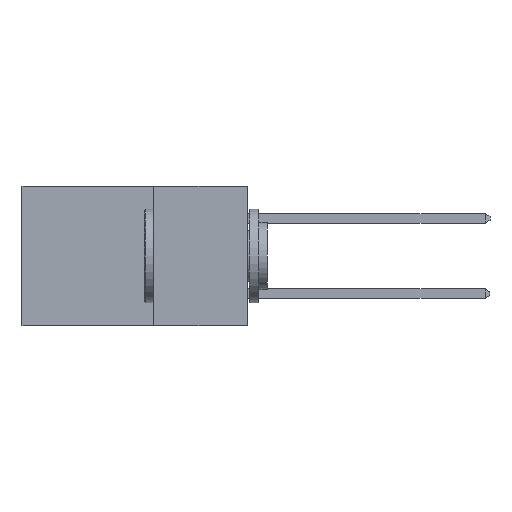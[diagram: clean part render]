
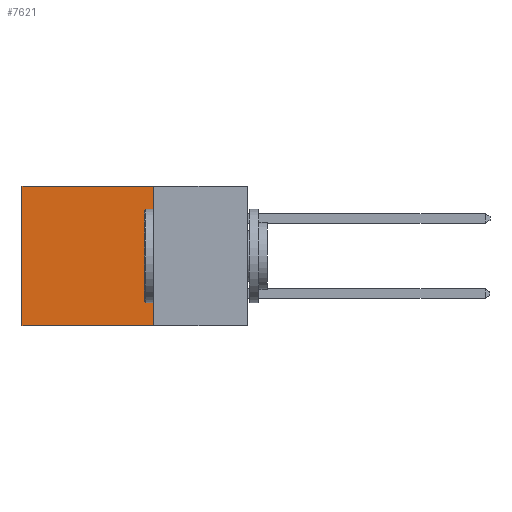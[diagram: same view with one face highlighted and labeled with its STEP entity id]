
A CAD part, left-side view. The second image highlights one B-rep face of the part: STEP entity #7621.
In plain terms, the highlighted planar face has unit normal (-1, 0, 0).
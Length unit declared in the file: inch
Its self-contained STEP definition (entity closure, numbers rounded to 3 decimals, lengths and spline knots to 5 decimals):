
#646 = EDGE_CURVE ( 'NONE', #6985, #10726, #9154, .T. ) ;
#1405 = VERTEX_POINT ( 'NONE', #12467 ) ;
#1589 = DIRECTION ( 'NONE',  ( 1., 0., 0. ) ) ;
#2355 = ORIENTED_EDGE ( 'NONE', *, *, #13315, .F. ) ;
#2408 = CARTESIAN_POINT ( 'NONE',  ( 0.298, 0.25, -0.37 ) ) ;
#2529 = CARTESIAN_POINT ( 'NONE',  ( 0.298, 0.25, 0. ) ) ;
#3327 = CARTESIAN_POINT ( 'NONE',  ( 0.298, 0.25, -0.37 ) ) ;
#3564 = VECTOR ( 'NONE', #13073, 39.37008 ) ;
#3726 = DIRECTION ( 'NONE',  ( 0., 1., 0. ) ) ;
#3819 = CARTESIAN_POINT ( 'NONE',  ( 0.298, 0.6, 0. ) ) ;
#4209 = FACE_OUTER_BOUND ( 'NONE', #15264, .T. ) ;
#4292 = AXIS2_PLACEMENT_3D ( 'NONE', #9465, #1589, #10846 ) ;
#5251 = DIRECTION ( 'NONE',  ( 0., 1., 0. ) ) ;
#6780 = PLANE ( 'NONE',  #4292 ) ;
#6985 = VERTEX_POINT ( 'NONE', #10686 ) ;
#7181 = VERTEX_POINT ( 'NONE', #3327 ) ;
#7621 = ADVANCED_FACE ( 'NONE', ( #4209 ), #6780, .F. ) ;
#7692 = CARTESIAN_POINT ( 'NONE',  ( 0.298, 0.25, 0. ) ) ;
#9154 = LINE ( 'NONE', #7692, #11916 ) ;
#9281 = LINE ( 'NONE', #2529, #3564 ) ;
#9465 = CARTESIAN_POINT ( 'NONE',  ( 0.298, 0.25, 0. ) ) ;
#10109 = VECTOR ( 'NONE', #3726, 39.37008 ) ;
#10428 = ORIENTED_EDGE ( 'NONE', *, *, #646, .T. ) ;
#10568 = LINE ( 'NONE', #2408, #10109 ) ;
#10686 = CARTESIAN_POINT ( 'NONE',  ( 0.298, 0.25, 0. ) ) ;
#10726 = VERTEX_POINT ( 'NONE', #14466 ) ;
#10846 = DIRECTION ( 'NONE',  ( 0., 0., -1. ) ) ;
#11916 = VECTOR ( 'NONE', #5251, 39.37008 ) ;
#12467 = CARTESIAN_POINT ( 'NONE',  ( 0.298, 0.6, -0.37 ) ) ;
#13050 = DIRECTION ( 'NONE',  ( 0., 0., -1. ) ) ;
#13073 = DIRECTION ( 'NONE',  ( 0., 0., -1. ) ) ;
#13243 = EDGE_CURVE ( 'NONE', #7181, #1405, #10568, .T. ) ;
#13315 = EDGE_CURVE ( 'NONE', #6985, #7181, #9281, .T. ) ;
#13478 = ORIENTED_EDGE ( 'NONE', *, *, #14013, .T. ) ;
#14013 = EDGE_CURVE ( 'NONE', #10726, #1405, #15948, .T. ) ;
#14342 = ORIENTED_EDGE ( 'NONE', *, *, #13243, .F. ) ;
#14466 = CARTESIAN_POINT ( 'NONE',  ( 0.298, 0.6, 0. ) ) ;
#15264 = EDGE_LOOP ( 'NONE', ( #13478, #14342, #2355, #10428 ) ) ;
#15523 = VECTOR ( 'NONE', #13050, 39.37008 ) ;
#15948 = LINE ( 'NONE', #3819, #15523 ) ;
